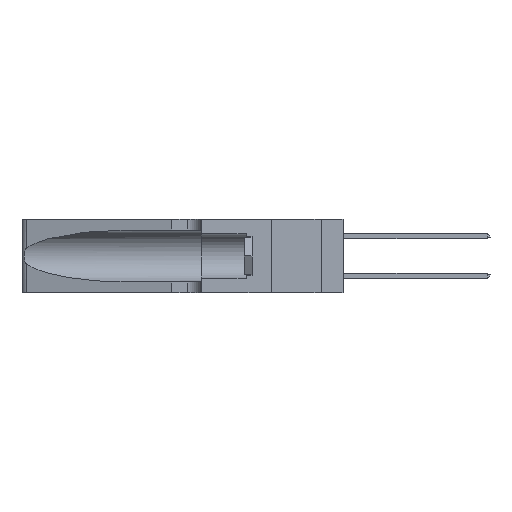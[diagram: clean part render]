
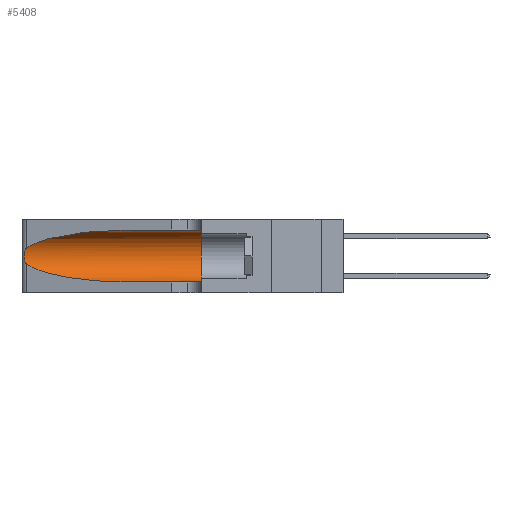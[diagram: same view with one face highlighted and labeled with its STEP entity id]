
A CAD part, left-side view. The second image highlights one B-rep face of the part: STEP entity #5408.
In plain terms, the highlighted cylindrical face has radius 3.308 mm (diameter 6.617 mm), a partial arc.
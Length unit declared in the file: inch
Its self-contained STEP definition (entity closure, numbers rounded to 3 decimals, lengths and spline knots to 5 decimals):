
#800 = CARTESIAN_POINT ( 'NONE',  ( 0.25787, 1.23484, 0.2124 ) ) ;
#1385 = DIRECTION ( 'NONE',  ( 0., 0., 1. ) ) ;
#1418 = CARTESIAN_POINT ( 'NONE',  ( 0.2373, 1.15595, 0.08982 ) ) ;
#4637 = CARTESIAN_POINT ( 'NONE',  ( 0.26018, 1.23835, 0.19895 ) ) ;
#5408 = ADVANCED_FACE ( 'NONE', ( #7961 ), #47186, .F. ) ;
#6689 = AXIS2_PLACEMENT_3D ( 'NONE', #25072, #13582, #28886 ) ;
#6855 = VERTEX_POINT ( 'NONE', #48647 ) ;
#7961 = FACE_OUTER_BOUND ( 'NONE', #24840, .T. ) ;
#8615 = CARTESIAN_POINT ( 'NONE',  ( 0.26075, 1.23896, 0.178 ) ) ;
#8956 = CARTESIAN_POINT ( 'NONE',  ( 0.1305, 0.72297, 0.31525 ) ) ;
#9562 = VECTOR ( 'NONE', #35038, 39.37008 ) ;
#9830 = CARTESIAN_POINT ( 'NONE',  ( 0.25487, 1.22718, 0.22369 ) ) ;
#12587 = CARTESIAN_POINT ( 'NONE',  ( 0.25856, 1.23593, 0.16098 ) ) ;
#13238 = CARTESIAN_POINT ( 'NONE',  ( 0.18966, 0.96281, 0.05475 ) ) ;
#13256 = VERTEX_POINT ( 'NONE', #44913 ) ;
#13582 = DIRECTION ( 'NONE',  ( 0., -1., 0. ) ) ;
#15172 = CARTESIAN_POINT ( 'NONE',  ( 0.1305, 0.35, 0.05475 ) ) ;
#16281 = CARTESIAN_POINT ( 'NONE',  ( 0.25487, 1.22718, 0.22369 ) ) ;
#16440 = CARTESIAN_POINT ( 'NONE',  ( 0.25639, 1.23186, 0.15144 ) ) ;
#19761 = ORIENTED_EDGE ( 'NONE', *, *, #27246, .T. ) ;
#20135 = CARTESIAN_POINT ( 'NONE',  ( 0.25555, 1.22994, 0.2215 ) ) ;
#20286 = CARTESIAN_POINT ( 'NONE',  ( 0.25487, 1.22718, 0.14631 ) ) ;
#20891 = EDGE_CURVE ( 'NONE', #22800, #13256, #40892, .T. ) ;
#21057 = VERTEX_POINT ( 'NONE', #33697 ) ;
#21285 = CARTESIAN_POINT ( 'NONE',  ( 0.18966, 0.96281, 0.31525 ) ) ;
#22107 = ORIENTED_EDGE ( 'NONE', *, *, #42940, .T. ) ;
#22800 = VERTEX_POINT ( 'NONE', #39438 ) ;
#23940 = CARTESIAN_POINT ( 'NONE',  ( 0.25639, 1.23184, 0.21858 ) ) ;
#24512 = DIRECTION ( 'NONE',  ( 0., 1., 0. ) ) ;
#24596 = EDGE_CURVE ( 'NONE', #21057, #38172, #39905, .T. ) ;
#24840 = EDGE_LOOP ( 'NONE', ( #19761, #39799, #22107, #46263, #29701, #41897 ) ) ;
#25072 = CARTESIAN_POINT ( 'NONE',  ( 0.1305, 1.61858, 0.185 ) ) ;
#25274 = B_SPLINE_CURVE_WITH_KNOTS ( 'NONE', 3,
 ( #16281, #20135, #23940, #800, #27769, #4637, #31545, #8615, #35320, #12587, #39093, #16440, #42872, #20286 ),
 .UNSPECIFIED., .F., .F.,
 ( 4, 2, 2, 2, 2, 2, 4 ),
 ( 0., 0.00027, 0.00053, 0.00107, 0.0016, 0.00187, 0.00214 ),
 .UNSPECIFIED. ) ;
#27246 = EDGE_CURVE ( 'NONE', #22800, #41311, #34057, .T. ) ;
#27769 = CARTESIAN_POINT ( 'NONE',  ( 0.25854, 1.2359, 0.20912 ) ) ;
#28886 = DIRECTION ( 'NONE',  ( 0., 0., -1. ) ) ;
#29701 = ORIENTED_EDGE ( 'NONE', *, *, #32644, .F. ) ;
#30663 = CARTESIAN_POINT ( 'NONE',  ( 0.25487, 1.22718, 0.22369 ) ) ;
#31279 = CARTESIAN_POINT ( 'NONE',  ( 0.1305, 1.61858, 0.05475 ) ) ;
#31545 = CARTESIAN_POINT ( 'NONE',  ( 0.26075, 1.23896, 0.19203 ) ) ;
#31582 = CIRCLE ( 'NONE', #34063, 0.13025 ) ;
#32157 = CARTESIAN_POINT ( 'NONE',  ( 0.25487, 1.22718, 0.14631 ) ) ;
#32644 = EDGE_CURVE ( 'NONE', #13256, #38172, #31582, .T. ) ;
#32717 = CARTESIAN_POINT ( 'NONE',  ( 0.2373, 1.15595, 0.28018 ) ) ;
#33697 = CARTESIAN_POINT ( 'NONE',  ( 0.1305, 0.72297, 0.05475 ) ) ;
#34057 =( BOUNDED_CURVE ( )  B_SPLINE_CURVE ( 3, ( #8956, #21285, #32717, #9830 ),
 .UNSPECIFIED., .F., .T. ) 
 B_SPLINE_CURVE_WITH_KNOTS ( ( 4, 4 ),
 ( 1.5708, 2.84003 ),
 .UNSPECIFIED. ) 
 CURVE ( )  GEOMETRIC_REPRESENTATION_ITEM ( )  RATIONAL_B_SPLINE_CURVE ( ( 1., 0.87, 0.87, 1. ) ) 
 REPRESENTATION_ITEM ( '' )  );
#34063 = AXIS2_PLACEMENT_3D ( 'NONE', #47064, #24512, #1385 ) ;
#35038 = DIRECTION ( 'NONE',  ( 0., -1., 0. ) ) ;
#35320 = CARTESIAN_POINT ( 'NONE',  ( 0.26017, 1.23833, 0.17102 ) ) ;
#36619 = CARTESIAN_POINT ( 'NONE',  ( 0.1305, 1.61858, 0.31525 ) ) ;
#38172 = VERTEX_POINT ( 'NONE', #15172 ) ;
#38391 = EDGE_CURVE ( 'NONE', #41311, #6855, #25274, .T. ) ;
#39093 = CARTESIAN_POINT ( 'NONE',  ( 0.25789, 1.23486, 0.15765 ) ) ;
#39438 = CARTESIAN_POINT ( 'NONE',  ( 0.1305, 0.72297, 0.31525 ) ) ;
#39697 = CARTESIAN_POINT ( 'NONE',  ( 0.1305, 0.72297, 0.05475 ) ) ;
#39799 = ORIENTED_EDGE ( 'NONE', *, *, #38391, .T. ) ;
#39905 = LINE ( 'NONE', #31279, #9562 ) ;
#40408 = DIRECTION ( 'NONE',  ( 0., -1., 0. ) ) ;
#40892 = LINE ( 'NONE', #36619, #45005 ) ;
#41311 = VERTEX_POINT ( 'NONE', #30663 ) ;
#41897 = ORIENTED_EDGE ( 'NONE', *, *, #20891, .F. ) ;
#42872 = CARTESIAN_POINT ( 'NONE',  ( 0.25555, 1.22993, 0.14849 ) ) ;
#42940 = EDGE_CURVE ( 'NONE', #6855, #21057, #47896, .T. ) ;
#44913 = CARTESIAN_POINT ( 'NONE',  ( 0.1305, 0.35, 0.31525 ) ) ;
#45005 = VECTOR ( 'NONE', #40408, 39.37008 ) ;
#46263 = ORIENTED_EDGE ( 'NONE', *, *, #24596, .T. ) ;
#47064 = CARTESIAN_POINT ( 'NONE',  ( 0.1305, 0.35, 0.185 ) ) ;
#47186 = CYLINDRICAL_SURFACE ( 'NONE', #6689, 0.13025 ) ;
#47896 =( BOUNDED_CURVE ( )  B_SPLINE_CURVE ( 3, ( #32157, #1418, #13238, #39697 ),
 .UNSPECIFIED., .F., .F. ) 
 B_SPLINE_CURVE_WITH_KNOTS ( ( 4, 4 ),
 ( 3.44316, 4.71239 ),
 .UNSPECIFIED. ) 
 CURVE ( )  GEOMETRIC_REPRESENTATION_ITEM ( )  RATIONAL_B_SPLINE_CURVE ( ( 1., 0.87, 0.87, 1. ) ) 
 REPRESENTATION_ITEM ( '' )  );
#48647 = CARTESIAN_POINT ( 'NONE',  ( 0.25487, 1.22718, 0.14631 ) ) ;
